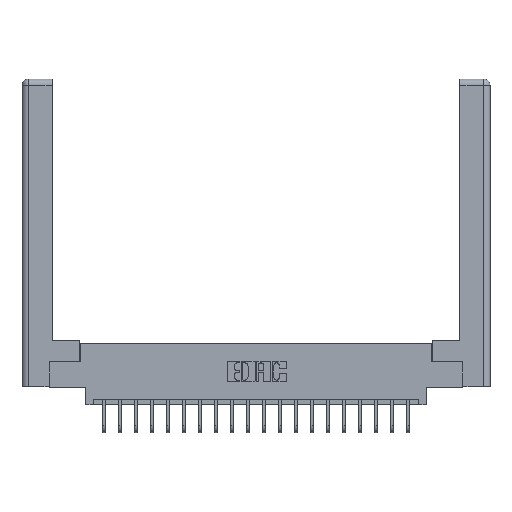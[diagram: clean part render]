
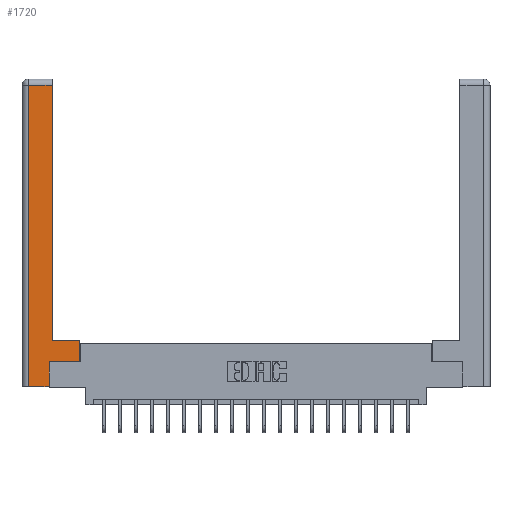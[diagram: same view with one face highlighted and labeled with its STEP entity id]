
A CAD part, top view. The second image highlights one B-rep face of the part: STEP entity #1720.
In plain terms, the highlighted planar face has unit normal (0, 0, 1).
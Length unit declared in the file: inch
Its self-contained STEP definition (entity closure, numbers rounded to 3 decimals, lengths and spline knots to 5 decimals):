
#378 = DIRECTION ( 'NONE',  ( 0., -1., 0. ) ) ;
#906 = ORIENTED_EDGE ( 'NONE', *, *, #9985, .T. ) ;
#1501 = ORIENTED_EDGE ( 'NONE', *, *, #9869, .T. ) ;
#1720 = ADVANCED_FACE ( 'NONE', ( #11330 ), #11265, .F. ) ;
#2140 = CARTESIAN_POINT ( 'NONE',  ( 0.295, 2.94, 0. ) ) ;
#2634 = EDGE_CURVE ( 'NONE', #16420, #5441, #6922, .T. ) ;
#2799 = LINE ( 'NONE', #3922, #5285 ) ;
#2914 = VECTOR ( 'NONE', #12042, 39.37008 ) ;
#2917 = EDGE_LOOP ( 'NONE', ( #17603, #16478, #7853, #6797, #4729, #1501, #16980, #906 ) ) ;
#3336 = CARTESIAN_POINT ( 'NONE',  ( 0.265, 0., 0. ) ) ;
#3774 = VECTOR ( 'NONE', #17269, 39.37008 ) ;
#3922 = CARTESIAN_POINT ( 'NONE',  ( 0.565, 0.245, 0. ) ) ;
#4249 = LINE ( 'NONE', #4470, #19693 ) ;
#4443 = CARTESIAN_POINT ( 'NONE',  ( 0.565, 0.45, 0. ) ) ;
#4470 = CARTESIAN_POINT ( 'NONE',  ( 0.265, 0.245, 0. ) ) ;
#4729 = ORIENTED_EDGE ( 'NONE', *, *, #10361, .T. ) ;
#4908 = VERTEX_POINT ( 'NONE', #10982 ) ;
#5166 = CARTESIAN_POINT ( 'NONE',  ( 0.0615, 0., 0. ) ) ;
#5285 = VECTOR ( 'NONE', #7202, 39.37008 ) ;
#5441 = VERTEX_POINT ( 'NONE', #3336 ) ;
#5855 = LINE ( 'NONE', #18651, #11351 ) ;
#5930 = CARTESIAN_POINT ( 'NONE',  ( 0.295, 0.45, 0. ) ) ;
#6208 = DIRECTION ( 'NONE',  ( 1., 0., 0. ) ) ;
#6486 = EDGE_CURVE ( 'NONE', #17522, #16873, #12862, .T. ) ;
#6797 = ORIENTED_EDGE ( 'NONE', *, *, #2634, .T. ) ;
#6922 = LINE ( 'NONE', #15857, #20097 ) ;
#7202 = DIRECTION ( 'NONE',  ( 1., 0., 0. ) ) ;
#7559 = VERTEX_POINT ( 'NONE', #9977 ) ;
#7853 = ORIENTED_EDGE ( 'NONE', *, *, #11926, .T. ) ;
#8374 = CARTESIAN_POINT ( 'NONE',  ( 0., 0., 0. ) ) ;
#8465 = VECTOR ( 'NONE', #378, 39.37008 ) ;
#8667 = VECTOR ( 'NONE', #10217, 39.37008 ) ;
#8981 = LINE ( 'NONE', #5166, #8465 ) ;
#9200 = AXIS2_PLACEMENT_3D ( 'NONE', #8374, #12968, #17852 ) ;
#9869 = EDGE_CURVE ( 'NONE', #13526, #17522, #2799, .T. ) ;
#9977 = CARTESIAN_POINT ( 'NONE',  ( 0.295, 0.45, 0. ) ) ;
#9985 = EDGE_CURVE ( 'NONE', #16873, #7559, #18942, .T. ) ;
#10217 = DIRECTION ( 'NONE',  ( -1., 0., 0. ) ) ;
#10361 = EDGE_CURVE ( 'NONE', #5441, #13526, #4249, .T. ) ;
#10982 = CARTESIAN_POINT ( 'NONE',  ( 0.0615, 2.94, 0. ) ) ;
#11265 = PLANE ( 'NONE',  #9200 ) ;
#11330 = FACE_OUTER_BOUND ( 'NONE', #2917, .T. ) ;
#11351 = VECTOR ( 'NONE', #17081, 39.37008 ) ;
#11692 = CARTESIAN_POINT ( 'NONE',  ( 0.565, 0.45, 0. ) ) ;
#11926 = EDGE_CURVE ( 'NONE', #4908, #16420, #8981, .T. ) ;
#12013 = CARTESIAN_POINT ( 'NONE',  ( 0.0615, 0., 0. ) ) ;
#12042 = DIRECTION ( 'NONE',  ( 0., 1., 0. ) ) ;
#12814 = EDGE_CURVE ( 'NONE', #15380, #4908, #19863, .T. ) ;
#12862 = LINE ( 'NONE', #11692, #2914 ) ;
#12968 = DIRECTION ( 'NONE',  ( 0., 0., -1. ) ) ;
#13526 = VERTEX_POINT ( 'NONE', #19840 ) ;
#14627 = CARTESIAN_POINT ( 'NONE',  ( 0.565, 0.245, 0. ) ) ;
#15380 = VERTEX_POINT ( 'NONE', #2140 ) ;
#15857 = CARTESIAN_POINT ( 'NONE',  ( 0.265, 0., 0. ) ) ;
#16420 = VERTEX_POINT ( 'NONE', #12013 ) ;
#16478 = ORIENTED_EDGE ( 'NONE', *, *, #12814, .T. ) ;
#16873 = VERTEX_POINT ( 'NONE', #4443 ) ;
#16980 = ORIENTED_EDGE ( 'NONE', *, *, #6486, .T. ) ;
#17081 = DIRECTION ( 'NONE',  ( 0., 1., 0. ) ) ;
#17269 = DIRECTION ( 'NONE',  ( -1., 0., 0. ) ) ;
#17522 = VERTEX_POINT ( 'NONE', #14627 ) ;
#17603 = ORIENTED_EDGE ( 'NONE', *, *, #18201, .T. ) ;
#17852 = DIRECTION ( 'NONE',  ( -1., 0., 0. ) ) ;
#18201 = EDGE_CURVE ( 'NONE', #7559, #15380, #5855, .T. ) ;
#18651 = CARTESIAN_POINT ( 'NONE',  ( 0.295, 3., 0. ) ) ;
#18942 = LINE ( 'NONE', #5930, #3774 ) ;
#19458 = CARTESIAN_POINT ( 'NONE',  ( 0.0615, 2.94, 0. ) ) ;
#19693 = VECTOR ( 'NONE', #20462, 39.37008 ) ;
#19840 = CARTESIAN_POINT ( 'NONE',  ( 0.265, 0.245, 0. ) ) ;
#19863 = LINE ( 'NONE', #19458, #8667 ) ;
#20097 = VECTOR ( 'NONE', #6208, 39.37008 ) ;
#20462 = DIRECTION ( 'NONE',  ( 0., 1., 0. ) ) ;
